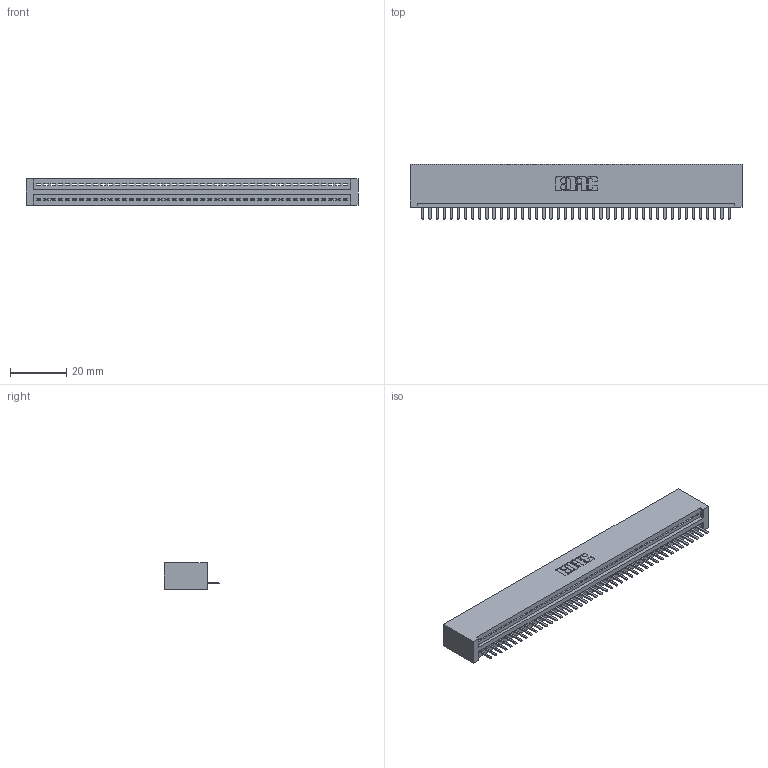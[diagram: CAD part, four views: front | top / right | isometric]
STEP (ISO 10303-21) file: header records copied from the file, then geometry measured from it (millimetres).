
FILE_DESCRIPTION (( 'STEP AP203' ), '1' );
FILE_NAME ('395-044-520-101.STEP', '2018-11-15T17:34:38', ( '' ), ( '' ), 'SwSTEP 2.0', 'SolidWorks 2016', '' );
FILE_SCHEMA (( 'CONFIG_CONTROL_DESIGN' ));
Length unit declared in the file: inch
Products named in the file (3): 345-292-001_345-293-120; 345 Part_No Mounting Lugs; 395-044-520-101
Assembly tree (45 placements, depth 2):
  395-044-520-101
    345 Part_No Mounting Lugs
    345-292-001_345-293-120  x44
Bounding box: 118.36 x 19.68 x 9.4 mm (x, y, z)
Volume: 11716.5 mm3; surface area: 15373.4 mm2
Topology: 45 solids, 45 shells, 2846 faces, 8413 edges, 5490 vertices
Faces by surface type: plane 1924, cylinder 922
Entity records: 32683 total; most frequent: CARTESIAN_POINT 5680, ORIENTED_EDGE 5646, DIRECTION 4939, EDGE_CURVE 2823, LINE 2519, VECTOR 2519, VERTEX_POINT 1878, AXIS2_PLACEMENT_3D 1210
